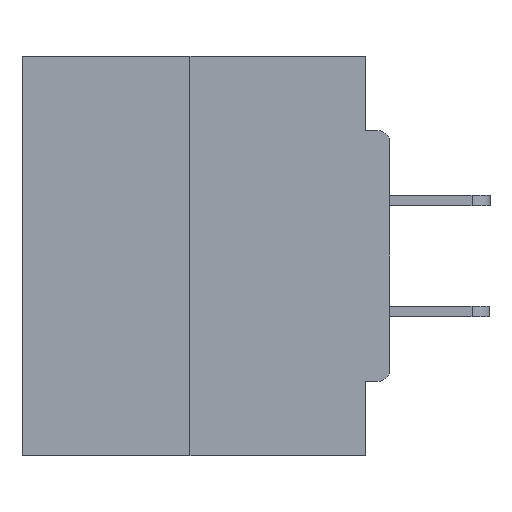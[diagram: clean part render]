
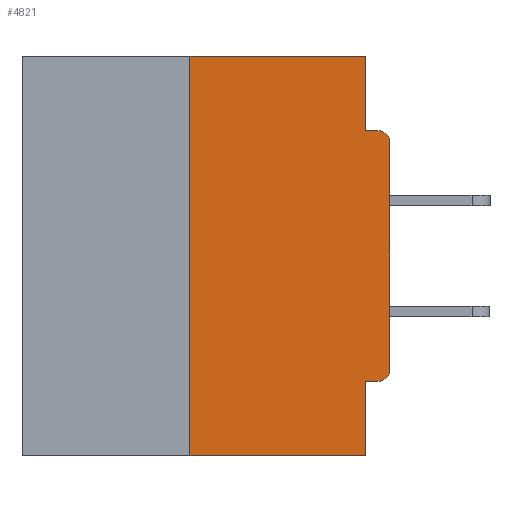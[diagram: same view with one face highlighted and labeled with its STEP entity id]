
A CAD part, left-side view. The second image highlights one B-rep face of the part: STEP entity #4821.
In plain terms, the highlighted planar face has unit normal (-1, 0, 0).
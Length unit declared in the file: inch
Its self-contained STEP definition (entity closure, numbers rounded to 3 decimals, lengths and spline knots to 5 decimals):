
#141 = CARTESIAN_POINT ( 'NONE',  ( 0., 0.015, -0.0935 ) ) ;
#808 = CARTESIAN_POINT ( 'NONE',  ( 0., 0.031, 0. ) ) ;
#843 = DIRECTION ( 'NONE',  ( 0., -1., 0. ) ) ;
#968 = LINE ( 'NONE', #25277, #9589 ) ;
#1523 = EDGE_CURVE ( 'NONE', #3568, #10321, #10061, .T. ) ;
#1738 = EDGE_CURVE ( 'NONE', #32421, #33698, #10892, .T. ) ;
#1932 = ORIENTED_EDGE ( 'NONE', *, *, #31110, .F. ) ;
#2410 = CARTESIAN_POINT ( 'NONE',  ( 0., 0.031, -0.5 ) ) ;
#3503 = CARTESIAN_POINT ( 'NONE',  ( 0., 0.46, 0. ) ) ;
#3568 = VERTEX_POINT ( 'NONE', #33811 ) ;
#3882 = EDGE_CURVE ( 'NONE', #22058, #10321, #12532, .T. ) ;
#4271 = FACE_OUTER_BOUND ( 'NONE', #9644, .T. ) ;
#4821 = ADVANCED_FACE ( 'NONE', ( #4271 ), #25090, .F. ) ;
#5710 = ORIENTED_EDGE ( 'NONE', *, *, #3882, .T. ) ;
#5916 = CARTESIAN_POINT ( 'NONE',  ( 0., 0.031, -0.5 ) ) ;
#6014 = CARTESIAN_POINT ( 'NONE',  ( 0., 0.015, -0.4065 ) ) ;
#6438 = EDGE_CURVE ( 'NONE', #13815, #17458, #33733, .T. ) ;
#6457 = ORIENTED_EDGE ( 'NONE', *, *, #9143, .F. ) ;
#7884 = AXIS2_PLACEMENT_3D ( 'NONE', #27892, #30549, #19241 ) ;
#8489 = VERTEX_POINT ( 'NONE', #20083 ) ;
#9143 = EDGE_CURVE ( 'NONE', #32970, #33698, #28150, .T. ) ;
#9377 = VECTOR ( 'NONE', #843, 39.37008 ) ;
#9422 = LINE ( 'NONE', #22024, #11152 ) ;
#9481 = VECTOR ( 'NONE', #31570, 39.37008 ) ;
#9577 = CARTESIAN_POINT ( 'NONE',  ( 0., 0.46, -0.5 ) ) ;
#9589 = VECTOR ( 'NONE', #25618, 39.37008 ) ;
#9644 = EDGE_LOOP ( 'NONE', ( #28531, #1932, #5710, #17388, #10375, #11832, #34575, #21815, #6457, #22227 ) ) ;
#10061 = LINE ( 'NONE', #5916, #22295 ) ;
#10321 = VERTEX_POINT ( 'NONE', #2410 ) ;
#10375 = ORIENTED_EDGE ( 'NONE', *, *, #33822, .F. ) ;
#10484 = DIRECTION ( 'NONE',  ( -1., 0., 0. ) ) ;
#10720 = CARTESIAN_POINT ( 'NONE',  ( 0., 0.015, -0.3915 ) ) ;
#10892 = CIRCLE ( 'NONE', #24874, 0.015 ) ;
#11152 = VECTOR ( 'NONE', #33325, 39.37008 ) ;
#11469 = VERTEX_POINT ( 'NONE', #6014 ) ;
#11832 = ORIENTED_EDGE ( 'NONE', *, *, #12336, .T. ) ;
#12011 = LINE ( 'NONE', #21124, #16823 ) ;
#12336 = EDGE_CURVE ( 'NONE', #11469, #8489, #13020, .T. ) ;
#12532 = LINE ( 'NONE', #9577, #19134 ) ;
#13020 = CIRCLE ( 'NONE', #30473, 0.015 ) ;
#13815 = VERTEX_POINT ( 'NONE', #16990 ) ;
#14238 = CARTESIAN_POINT ( 'NONE',  ( 0., 0., -0.0935 ) ) ;
#14793 = CARTESIAN_POINT ( 'NONE',  ( 0., 0.25, -0.5 ) ) ;
#14973 = CARTESIAN_POINT ( 'NONE',  ( 0., 0.25, 0. ) ) ;
#16395 = CARTESIAN_POINT ( 'NONE',  ( 0., 0.031, -0.0935 ) ) ;
#16823 = VECTOR ( 'NONE', #26983, 39.37008 ) ;
#16883 = LINE ( 'NONE', #14973, #9481 ) ;
#16990 = CARTESIAN_POINT ( 'NONE',  ( 0., 0.25, 0. ) ) ;
#17226 = DIRECTION ( 'NONE',  ( 0., -1., 0. ) ) ;
#17388 = ORIENTED_EDGE ( 'NONE', *, *, #1523, .F. ) ;
#17458 = VERTEX_POINT ( 'NONE', #808 ) ;
#18076 = CARTESIAN_POINT ( 'NONE',  ( 0., 0., -0.1085 ) ) ;
#19134 = VECTOR ( 'NONE', #20820, 39.37008 ) ;
#19241 = DIRECTION ( 'NONE',  ( 0., 0., -1. ) ) ;
#20083 = CARTESIAN_POINT ( 'NONE',  ( 0., 0., -0.3915 ) ) ;
#20820 = DIRECTION ( 'NONE',  ( 0., -1., 0. ) ) ;
#21124 = CARTESIAN_POINT ( 'NONE',  ( 0., 0.031, 0. ) ) ;
#21287 = EDGE_CURVE ( 'NONE', #8489, #32421, #9422, .T. ) ;
#21793 = DIRECTION ( 'NONE',  ( 0., 0., -1. ) ) ;
#21815 = ORIENTED_EDGE ( 'NONE', *, *, #1738, .T. ) ;
#22024 = CARTESIAN_POINT ( 'NONE',  ( 0., 0., 0. ) ) ;
#22058 = VERTEX_POINT ( 'NONE', #14793 ) ;
#22227 = ORIENTED_EDGE ( 'NONE', *, *, #32501, .F. ) ;
#22295 = VECTOR ( 'NONE', #31759, 39.37008 ) ;
#24874 = AXIS2_PLACEMENT_3D ( 'NONE', #30300, #35888, #21793 ) ;
#25090 = PLANE ( 'NONE',  #7884 ) ;
#25277 = CARTESIAN_POINT ( 'NONE',  ( 0., 0., -0.4065 ) ) ;
#25618 = DIRECTION ( 'NONE',  ( 0., 1., 0. ) ) ;
#26983 = DIRECTION ( 'NONE',  ( 0., 0., -1. ) ) ;
#27643 = VECTOR ( 'NONE', #17226, 39.37008 ) ;
#27892 = CARTESIAN_POINT ( 'NONE',  ( 0., 0.46, 0. ) ) ;
#28150 = LINE ( 'NONE', #14238, #9377 ) ;
#28531 = ORIENTED_EDGE ( 'NONE', *, *, #6438, .F. ) ;
#30300 = CARTESIAN_POINT ( 'NONE',  ( 0., 0.015, -0.1085 ) ) ;
#30473 = AXIS2_PLACEMENT_3D ( 'NONE', #10720, #10484, #35602 ) ;
#30549 = DIRECTION ( 'NONE',  ( 1., 0., 0. ) ) ;
#31110 = EDGE_CURVE ( 'NONE', #22058, #13815, #16883, .T. ) ;
#31570 = DIRECTION ( 'NONE',  ( 0., 0., 1. ) ) ;
#31759 = DIRECTION ( 'NONE',  ( 0., 0., -1. ) ) ;
#32421 = VERTEX_POINT ( 'NONE', #18076 ) ;
#32501 = EDGE_CURVE ( 'NONE', #17458, #32970, #12011, .T. ) ;
#32970 = VERTEX_POINT ( 'NONE', #16395 ) ;
#33325 = DIRECTION ( 'NONE',  ( 0., 0., 1. ) ) ;
#33698 = VERTEX_POINT ( 'NONE', #141 ) ;
#33733 = LINE ( 'NONE', #3503, #27643 ) ;
#33811 = CARTESIAN_POINT ( 'NONE',  ( 0., 0.031, -0.4065 ) ) ;
#33822 = EDGE_CURVE ( 'NONE', #11469, #3568, #968, .T. ) ;
#34575 = ORIENTED_EDGE ( 'NONE', *, *, #21287, .T. ) ;
#35602 = DIRECTION ( 'NONE',  ( 0., 0., -1. ) ) ;
#35888 = DIRECTION ( 'NONE',  ( -1., 0., 0. ) ) ;
